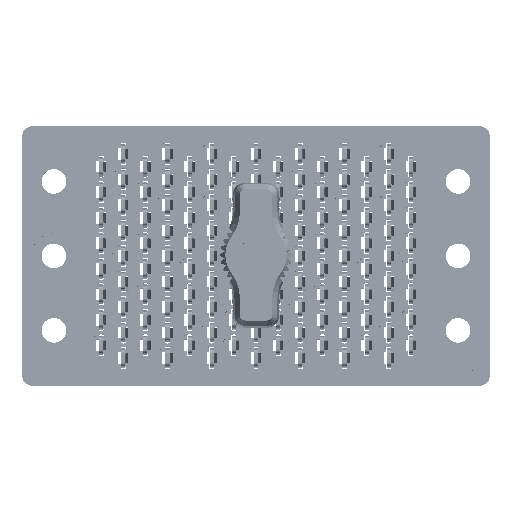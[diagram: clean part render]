
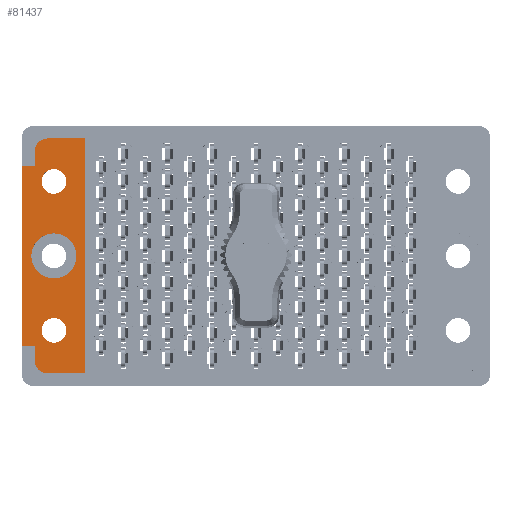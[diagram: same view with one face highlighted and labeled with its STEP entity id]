
A CAD part, top view. The second image highlights one B-rep face of the part: STEP entity #81437.
In plain terms, the highlighted planar face has unit normal (0, 0, 1).
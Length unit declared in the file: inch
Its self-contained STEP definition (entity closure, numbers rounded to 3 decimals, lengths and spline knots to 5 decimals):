
#685 = DIRECTION ( 'NONE',  ( 0., 0., 1. ) ) ;
#1031 = CARTESIAN_POINT ( 'NONE',  ( -1.1875, 0.4375, -0.117 ) ) ;
#1617 = CARTESIAN_POINT ( 'NONE',  ( -1.115, 0.4375, -0.117 ) ) ;
#1683 = DIRECTION ( 'NONE',  ( 1., 0., 0. ) ) ;
#2063 = CIRCLE ( 'NONE', #36705, 0.0725 ) ;
#2746 = FACE_BOUND ( 'NONE', #71502, .T. ) ;
#2841 = EDGE_LOOP ( 'NONE', ( #80532, #10138, #13602, #100320, #9465, #50410, #25692, #95247, #64623, #49171 ) ) ;
#4036 = VERTEX_POINT ( 'NONE', #31174 ) ;
#4775 = VECTOR ( 'NONE', #72162, 39.37008 ) ;
#6040 = CARTESIAN_POINT ( 'NONE',  ( -1.3, 0., -0.117 ) ) ;
#6758 = CARTESIAN_POINT ( 'NONE',  ( 0., -0.69, -0.117 ) ) ;
#7326 = CARTESIAN_POINT ( 'NONE',  ( -1.3, -0.5285, -0.117 ) ) ;
#7846 = LINE ( 'NONE', #6758, #44812 ) ;
#9287 = EDGE_LOOP ( 'NONE', ( #76414, #33857 ) ) ;
#9465 = ORIENTED_EDGE ( 'NONE', *, *, #77844, .T. ) ;
#10035 = EDGE_CURVE ( 'NONE', #4036, #42920, #7846, .T. ) ;
#10138 = ORIENTED_EDGE ( 'NONE', *, *, #23944, .T. ) ;
#10814 = CARTESIAN_POINT ( 'NONE',  ( -1.1875, 0., -0.117 ) ) ;
#11422 = FACE_BOUND ( 'NONE', #9287, .T. ) ;
#12967 = DIRECTION ( 'NONE',  ( -1., 0., 0. ) ) ;
#13602 = ORIENTED_EDGE ( 'NONE', *, *, #54274, .T. ) ;
#13640 = CARTESIAN_POINT ( 'NONE',  ( -1.1875, -0.4375, -0.117 ) ) ;
#14178 = CARTESIAN_POINT ( 'NONE',  ( -1.1875, -0.4375, -0.117 ) ) ;
#14548 = VERTEX_POINT ( 'NONE', #1617 ) ;
#15448 = CARTESIAN_POINT ( 'NONE',  ( -1.005, 0.69, -0.117 ) ) ;
#16398 = VECTOR ( 'NONE', #98378, 39.37008 ) ;
#16670 = CARTESIAN_POINT ( 'NONE',  ( -1.26, 0.4375, -0.117 ) ) ;
#17076 = CARTESIAN_POINT ( 'NONE',  ( -1.225, 0.615, -0.117 ) ) ;
#17610 = EDGE_CURVE ( 'NONE', #100048, #46769, #103659, .T. ) ;
#18305 = CIRCLE ( 'NONE', #61554, 0.075 ) ;
#18489 = DIRECTION ( 'NONE',  ( 0., 0., 1. ) ) ;
#21327 = CARTESIAN_POINT ( 'NONE',  ( -1.375, -0.5285, -0.117 ) ) ;
#22435 = AXIS2_PLACEMENT_3D ( 'NONE', #1031, #42732, #34575 ) ;
#22839 = DIRECTION ( 'NONE',  ( 0., 0., 1. ) ) ;
#23944 = EDGE_CURVE ( 'NONE', #35098, #71282, #67399, .T. ) ;
#25692 = ORIENTED_EDGE ( 'NONE', *, *, #17610, .T. ) ;
#26659 = CARTESIAN_POINT ( 'NONE',  ( -1.1875, 0., -0.117 ) ) ;
#28670 = EDGE_CURVE ( 'NONE', #4036, #33743, #86031, .T. ) ;
#30038 = VERTEX_POINT ( 'NONE', #106624 ) ;
#30724 = CARTESIAN_POINT ( 'NONE',  ( 0., 0.69, -0.117 ) ) ;
#31113 = LINE ( 'NONE', #64208, #16398 ) ;
#31174 = CARTESIAN_POINT ( 'NONE',  ( -1.005, -0.69, -0.117 ) ) ;
#31485 = DIRECTION ( 'NONE',  ( 0., 0., 1. ) ) ;
#33329 = LINE ( 'NONE', #98986, #34190 ) ;
#33665 = CARTESIAN_POINT ( 'NONE',  ( -1.3, -0.615, -0.117 ) ) ;
#33743 = VERTEX_POINT ( 'NONE', #15448 ) ;
#33763 = DIRECTION ( 'NONE',  ( 1., 0., 0. ) ) ;
#33857 = ORIENTED_EDGE ( 'NONE', *, *, #45496, .F. ) ;
#34190 = VECTOR ( 'NONE', #66945, 39.37008 ) ;
#34575 = DIRECTION ( 'NONE',  ( 1., 0., 0. ) ) ;
#35002 = AXIS2_PLACEMENT_3D ( 'NONE', #26659, #685, #101497 ) ;
#35098 = VERTEX_POINT ( 'NONE', #52806 ) ;
#35399 = EDGE_CURVE ( 'NONE', #69197, #104886, #81768, .T. ) ;
#36012 = EDGE_CURVE ( 'NONE', #82176, #30038, #95915, .T. ) ;
#36231 = CARTESIAN_POINT ( 'NONE',  ( -1.3, 0.5285, -0.117 ) ) ;
#36375 = CARTESIAN_POINT ( 'NONE',  ( -1.1875, 0.4375, -0.117 ) ) ;
#36705 = AXIS2_PLACEMENT_3D ( 'NONE', #14178, #31485, #97121 ) ;
#36972 = VECTOR ( 'NONE', #70275, 39.37008 ) ;
#39066 = DIRECTION ( 'NONE',  ( 1., 0., 0. ) ) ;
#39118 = VERTEX_POINT ( 'NONE', #16670 ) ;
#39315 = CARTESIAN_POINT ( 'NONE',  ( -1.225, -0.69, -0.117 ) ) ;
#39815 = DIRECTION ( 'NONE',  ( 1., 0., 0. ) ) ;
#40741 = EDGE_CURVE ( 'NONE', #104886, #69197, #84158, .T. ) ;
#41696 = DIRECTION ( 'NONE',  ( 0., 0., 1. ) ) ;
#42732 = DIRECTION ( 'NONE',  ( 0., 0., 1. ) ) ;
#42920 = VERTEX_POINT ( 'NONE', #39315 ) ;
#43079 = EDGE_CURVE ( 'NONE', #100048, #59059, #33329, .T. ) ;
#44163 = EDGE_LOOP ( 'NONE', ( #58367, #44965 ) ) ;
#44812 = VECTOR ( 'NONE', #65304, 39.37008 ) ;
#44965 = ORIENTED_EDGE ( 'NONE', *, *, #40741, .F. ) ;
#45496 = EDGE_CURVE ( 'NONE', #14548, #39118, #50138, .T. ) ;
#46769 = VERTEX_POINT ( 'NONE', #33665 ) ;
#49171 = ORIENTED_EDGE ( 'NONE', *, *, #28670, .T. ) ;
#50134 = AXIS2_PLACEMENT_3D ( 'NONE', #17076, #98954, #39815 ) ;
#50138 = CIRCLE ( 'NONE', #22435, 0.0725 ) ;
#50410 = ORIENTED_EDGE ( 'NONE', *, *, #43079, .F. ) ;
#50994 = CARTESIAN_POINT ( 'NONE',  ( -1.375, -0.7625, -0.117 ) ) ;
#52499 = VERTEX_POINT ( 'NONE', #89332 ) ;
#52806 = CARTESIAN_POINT ( 'NONE',  ( -1.225, 0.69, -0.117 ) ) ;
#53288 = AXIS2_PLACEMENT_3D ( 'NONE', #36375, #58664, #67887 ) ;
#54274 = EDGE_CURVE ( 'NONE', #71282, #82176, #31113, .T. ) ;
#54788 = ORIENTED_EDGE ( 'NONE', *, *, #89253, .F. ) ;
#58367 = ORIENTED_EDGE ( 'NONE', *, *, #35399, .F. ) ;
#58664 = DIRECTION ( 'NONE',  ( 0., 0., 1. ) ) ;
#59059 = VERTEX_POINT ( 'NONE', #21327 ) ;
#60049 = AXIS2_PLACEMENT_3D ( 'NONE', #50994, #18489, #1683 ) ;
#61119 = VECTOR ( 'NONE', #12967, 39.37008 ) ;
#61554 = AXIS2_PLACEMENT_3D ( 'NONE', #83135, #97822, #33763 ) ;
#64208 = CARTESIAN_POINT ( 'NONE',  ( -1.3, 0., -0.117 ) ) ;
#64401 = AXIS2_PLACEMENT_3D ( 'NONE', #13640, #22839, #39066 ) ;
#64623 = ORIENTED_EDGE ( 'NONE', *, *, #10035, .F. ) ;
#65304 = DIRECTION ( 'NONE',  ( -1., 0., 0. ) ) ;
#65406 = DIRECTION ( 'NONE',  ( -1., 0., 0. ) ) ;
#66885 = CARTESIAN_POINT ( 'NONE',  ( -1.375, 0.7625, -0.117 ) ) ;
#66945 = DIRECTION ( 'NONE',  ( -1., 0., 0. ) ) ;
#67399 = CIRCLE ( 'NONE', #50134, 0.075 ) ;
#67887 = DIRECTION ( 'NONE',  ( 1., 0., 0. ) ) ;
#69197 = VERTEX_POINT ( 'NONE', #98406 ) ;
#69347 = ORIENTED_EDGE ( 'NONE', *, *, #89366, .F. ) ;
#70275 = DIRECTION ( 'NONE',  ( 0., 1., 0. ) ) ;
#71282 = VERTEX_POINT ( 'NONE', #86341 ) ;
#71502 = EDGE_LOOP ( 'NONE', ( #54788, #69347 ) ) ;
#72162 = DIRECTION ( 'NONE',  ( 0., -1., 0. ) ) ;
#73620 = CARTESIAN_POINT ( 'NONE',  ( -1.115, -0.4375, -0.117 ) ) ;
#76414 = ORIENTED_EDGE ( 'NONE', *, *, #83194, .F. ) ;
#76937 = DIRECTION ( 'NONE',  ( 1., 0., 0. ) ) ;
#77018 = PLANE ( 'NONE',  #60049 ) ;
#77254 = EDGE_CURVE ( 'NONE', #33743, #35098, #106616, .T. ) ;
#77844 = EDGE_CURVE ( 'NONE', #30038, #59059, #98919, .T. ) ;
#78028 = CARTESIAN_POINT ( 'NONE',  ( 0., 0.5285, -0.117 ) ) ;
#78439 = CARTESIAN_POINT ( 'NONE',  ( -1.005, 0.7625, -0.117 ) ) ;
#78719 = VERTEX_POINT ( 'NONE', #73620 ) ;
#78800 = VECTOR ( 'NONE', #99981, 39.37008 ) ;
#78975 = AXIS2_PLACEMENT_3D ( 'NONE', #10814, #41696, #76937 ) ;
#80532 = ORIENTED_EDGE ( 'NONE', *, *, #77254, .T. ) ;
#81437 = ADVANCED_FACE ( 'NONE', ( #11422, #2746, #84621, #84082 ), #77018, .T. ) ;
#81768 = CIRCLE ( 'NONE', #35002, 0.1325 ) ;
#82176 = VERTEX_POINT ( 'NONE', #36231 ) ;
#83135 = CARTESIAN_POINT ( 'NONE',  ( -1.225, -0.615, -0.117 ) ) ;
#83194 = EDGE_CURVE ( 'NONE', #39118, #14548, #101767, .T. ) ;
#84082 = FACE_OUTER_BOUND ( 'NONE', #2841, .T. ) ;
#84158 = CIRCLE ( 'NONE', #78975, 0.1325 ) ;
#84621 = FACE_BOUND ( 'NONE', #44163, .T. ) ;
#86031 = LINE ( 'NONE', #78439, #36972 ) ;
#86341 = CARTESIAN_POINT ( 'NONE',  ( -1.3, 0.615, -0.117 ) ) ;
#89253 = EDGE_CURVE ( 'NONE', #52499, #78719, #99038, .T. ) ;
#89332 = CARTESIAN_POINT ( 'NONE',  ( -1.26, -0.4375, -0.117 ) ) ;
#89366 = EDGE_CURVE ( 'NONE', #78719, #52499, #2063, .T. ) ;
#94298 = VECTOR ( 'NONE', #65406, 39.37008 ) ;
#95247 = ORIENTED_EDGE ( 'NONE', *, *, #103616, .T. ) ;
#95915 = LINE ( 'NONE', #78028, #61119 ) ;
#97121 = DIRECTION ( 'NONE',  ( 1., 0., 0. ) ) ;
#97822 = DIRECTION ( 'NONE',  ( 0., 0., 1. ) ) ;
#98378 = DIRECTION ( 'NONE',  ( 0., -1., 0. ) ) ;
#98406 = CARTESIAN_POINT ( 'NONE',  ( -1.055, 0., -0.117 ) ) ;
#98919 = LINE ( 'NONE', #66885, #78800 ) ;
#98954 = DIRECTION ( 'NONE',  ( 0., 0., 1. ) ) ;
#98986 = CARTESIAN_POINT ( 'NONE',  ( 0., -0.5285, -0.117 ) ) ;
#99038 = CIRCLE ( 'NONE', #64401, 0.0725 ) ;
#99981 = DIRECTION ( 'NONE',  ( 0., -1., 0. ) ) ;
#100048 = VERTEX_POINT ( 'NONE', #7326 ) ;
#100320 = ORIENTED_EDGE ( 'NONE', *, *, #36012, .T. ) ;
#101497 = DIRECTION ( 'NONE',  ( 1., 0., 0. ) ) ;
#101767 = CIRCLE ( 'NONE', #53288, 0.0725 ) ;
#103616 = EDGE_CURVE ( 'NONE', #46769, #42920, #18305, .T. ) ;
#103659 = LINE ( 'NONE', #6040, #4775 ) ;
#104361 = CARTESIAN_POINT ( 'NONE',  ( -1.32, 0., -0.117 ) ) ;
#104886 = VERTEX_POINT ( 'NONE', #104361 ) ;
#106616 = LINE ( 'NONE', #30724, #94298 ) ;
#106624 = CARTESIAN_POINT ( 'NONE',  ( -1.375, 0.5285, -0.117 ) ) ;
